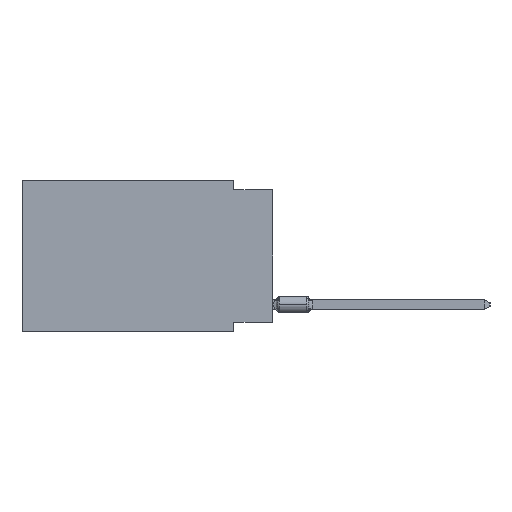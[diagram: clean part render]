
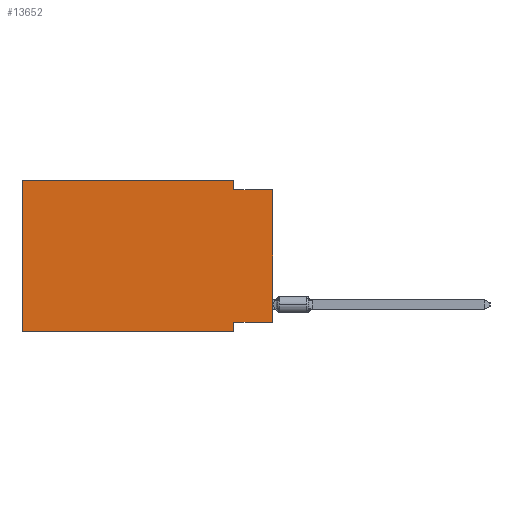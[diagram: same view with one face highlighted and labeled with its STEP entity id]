
A CAD part, left-side view. The second image highlights one B-rep face of the part: STEP entity #13652.
In plain terms, the highlighted planar face has unit normal (-1, 0, 0).
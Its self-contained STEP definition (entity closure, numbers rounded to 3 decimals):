
#40 = ORIENTED_EDGE ( 'NONE', *, *, #35929, .F. ) ;
#1477 = DIRECTION ( 'NONE',  ( 0., 0., 1. ) ) ;
#3718 = VERTEX_POINT ( 'NONE', #17191 ) ;
#3901 = CARTESIAN_POINT ( 'NONE',  ( 0., 16.383, -9.906 ) ) ;
#3927 = CARTESIAN_POINT ( 'NONE',  ( 0., 2.54, -9.906 ) ) ;
#4248 = LINE ( 'NONE', #3901, #9281 ) ;
#5719 = ORIENTED_EDGE ( 'NONE', *, *, #22537, .F. ) ;
#6141 = VECTOR ( 'NONE', #32284, 1000. ) ;
#6199 = DIRECTION ( 'NONE',  ( 0., 1., 0. ) ) ;
#6505 = VERTEX_POINT ( 'NONE', #62269 ) ;
#7932 = VECTOR ( 'NONE', #38507, 1000. ) ;
#8410 = EDGE_CURVE ( 'NONE', #60829, #50507, #12221, .T. ) ;
#9281 = VECTOR ( 'NONE', #20223, 1000. ) ;
#9395 = EDGE_CURVE ( 'NONE', #3718, #60829, #49381, .T. ) ;
#10255 = DIRECTION ( 'NONE',  ( 1., 0., 0. ) ) ;
#10604 = CARTESIAN_POINT ( 'NONE',  ( 0., 2.54, 0. ) ) ;
#10863 = ORIENTED_EDGE ( 'NONE', *, *, #9395, .F. ) ;
#11629 = LINE ( 'NONE', #33749, #66050 ) ;
#12221 = LINE ( 'NONE', #45919, #51949 ) ;
#13652 = ADVANCED_FACE ( 'NONE', ( #33077 ), #43240, .F. ) ;
#15697 = CARTESIAN_POINT ( 'NONE',  ( 0., 16.383, 0. ) ) ;
#17191 = CARTESIAN_POINT ( 'NONE',  ( 0., 2.54, 0. ) ) ;
#17707 = VERTEX_POINT ( 'NONE', #3927 ) ;
#18088 = DIRECTION ( 'NONE',  ( 0., 0., 1. ) ) ;
#20223 = DIRECTION ( 'NONE',  ( 0., -1., 0. ) ) ;
#21054 = LINE ( 'NONE', #54026, #30870 ) ;
#22356 = EDGE_LOOP ( 'NONE', ( #37003, #63527, #10863, #67186, #40, #39957, #34195, #5719 ) ) ;
#22537 = EDGE_CURVE ( 'NONE', #49335, #38913, #11629, .T. ) ;
#23224 = CARTESIAN_POINT ( 'NONE',  ( 0., 16.383, 0. ) ) ;
#23919 = CARTESIAN_POINT ( 'NONE',  ( 0., 0., -0.635 ) ) ;
#24302 = CARTESIAN_POINT ( 'NONE',  ( 0., 16.383, 0. ) ) ;
#28669 = LINE ( 'NONE', #24302, #48891 ) ;
#30870 = VECTOR ( 'NONE', #60880, 1000. ) ;
#31461 = EDGE_CURVE ( 'NONE', #6505, #17707, #4248, .T. ) ;
#32284 = DIRECTION ( 'NONE',  ( 0., -1., 0. ) ) ;
#32375 = DIRECTION ( 'NONE',  ( 0., 0., -1. ) ) ;
#33052 = VERTEX_POINT ( 'NONE', #23224 ) ;
#33077 = FACE_OUTER_BOUND ( 'NONE', #22356, .T. ) ;
#33749 = CARTESIAN_POINT ( 'NONE',  ( 0., 0., -9.271 ) ) ;
#34195 = ORIENTED_EDGE ( 'NONE', *, *, #66223, .F. ) ;
#34342 = DIRECTION ( 'NONE',  ( 0., -1., 0. ) ) ;
#35865 = CARTESIAN_POINT ( 'NONE',  ( 0., 2.54, -0.635 ) ) ;
#35929 = EDGE_CURVE ( 'NONE', #6505, #33052, #28669, .T. ) ;
#36786 = CARTESIAN_POINT ( 'NONE',  ( 0., 2.54, -9.271 ) ) ;
#37003 = ORIENTED_EDGE ( 'NONE', *, *, #69723, .T. ) ;
#38507 = DIRECTION ( 'NONE',  ( 0., 0., -1. ) ) ;
#38913 = VERTEX_POINT ( 'NONE', #36786 ) ;
#39957 = ORIENTED_EDGE ( 'NONE', *, *, #31461, .T. ) ;
#41682 = VECTOR ( 'NONE', #18088, 1000. ) ;
#43240 = PLANE ( 'NONE',  #46704 ) ;
#45919 = CARTESIAN_POINT ( 'NONE',  ( 0., 0., -0.635 ) ) ;
#46704 = AXIS2_PLACEMENT_3D ( 'NONE', #15697, #10255, #32375 ) ;
#48891 = VECTOR ( 'NONE', #1477, 1000. ) ;
#49335 = VERTEX_POINT ( 'NONE', #50836 ) ;
#49381 = LINE ( 'NONE', #10604, #7932 ) ;
#50348 = LINE ( 'NONE', #56872, #41682 ) ;
#50507 = VERTEX_POINT ( 'NONE', #23919 ) ;
#50836 = CARTESIAN_POINT ( 'NONE',  ( 0., 0., -9.271 ) ) ;
#51949 = VECTOR ( 'NONE', #34342, 1000. ) ;
#53314 = LINE ( 'NONE', #71060, #6141 ) ;
#54026 = CARTESIAN_POINT ( 'NONE',  ( 0., 2.54, -9.906 ) ) ;
#56872 = CARTESIAN_POINT ( 'NONE',  ( 0., 0., 0. ) ) ;
#60829 = VERTEX_POINT ( 'NONE', #35865 ) ;
#60880 = DIRECTION ( 'NONE',  ( 0., 0., -1. ) ) ;
#62269 = CARTESIAN_POINT ( 'NONE',  ( 0., 16.383, -9.906 ) ) ;
#63527 = ORIENTED_EDGE ( 'NONE', *, *, #8410, .F. ) ;
#66050 = VECTOR ( 'NONE', #6199, 1000. ) ;
#66223 = EDGE_CURVE ( 'NONE', #38913, #17707, #21054, .T. ) ;
#67186 = ORIENTED_EDGE ( 'NONE', *, *, #71381, .F. ) ;
#69723 = EDGE_CURVE ( 'NONE', #49335, #50507, #50348, .T. ) ;
#71060 = CARTESIAN_POINT ( 'NONE',  ( 0., 16.383, 0. ) ) ;
#71381 = EDGE_CURVE ( 'NONE', #33052, #3718, #53314, .T. ) ;
